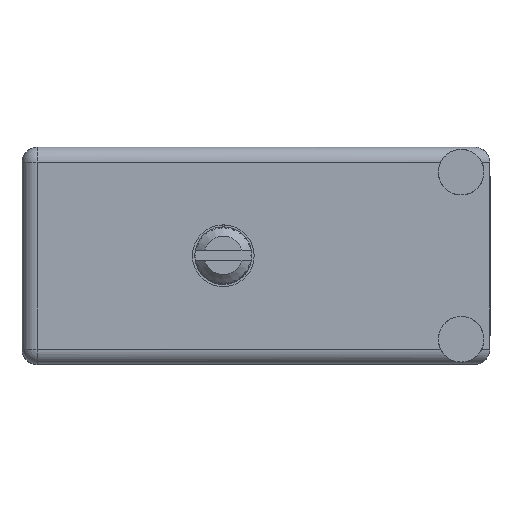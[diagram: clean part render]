
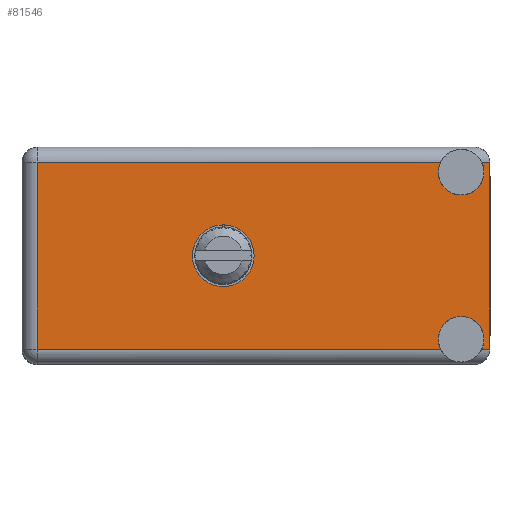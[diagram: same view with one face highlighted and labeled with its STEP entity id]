
A CAD part, top view. The second image highlights one B-rep face of the part: STEP entity #81546.
In plain terms, the highlighted face is planar.
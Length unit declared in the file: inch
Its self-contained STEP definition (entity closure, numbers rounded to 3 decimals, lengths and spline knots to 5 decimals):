
#1102 = EDGE_LOOP ( 'NONE', ( #109759, #47363 ) ) ;
#2539 = ORIENTED_EDGE ( 'NONE', *, *, #103446, .T. ) ;
#3104 = EDGE_CURVE ( 'NONE', #85294, #27077, #30411, .T. ) ;
#4047 = DIRECTION ( 'NONE',  ( 0., 1., 0. ) ) ;
#4627 = CARTESIAN_POINT ( 'NONE',  ( 1.37741, 0.906, -0.05 ) ) ;
#10379 = LINE ( 'NONE', #58055, #128065 ) ;
#10570 = VERTEX_POINT ( 'NONE', #101009 ) ;
#13580 = AXIS2_PLACEMENT_3D ( 'NONE', #35448, #127387, #113257 ) ;
#13898 = VERTEX_POINT ( 'NONE', #93714 ) ;
#14114 = LINE ( 'NONE', #29586, #66838 ) ;
#20758 = EDGE_CURVE ( 'NONE', #189943, #94466, #188819, .T. ) ;
#22841 = CARTESIAN_POINT ( 'NONE',  ( 1.445, 0.906, -0.0825 ) ) ;
#23525 = CARTESIAN_POINT ( 'NONE',  ( 0.6625, 0.906, -0.459 ) ) ;
#24242 = CARTESIAN_POINT ( 'NONE',  ( 0.05, 0.906, -0.05 ) ) ;
#24729 = AXIS2_PLACEMENT_3D ( 'NONE', #22841, #69061, #100625 ) ;
#26307 = DIRECTION ( 'NONE',  ( 0., 0., 1. ) ) ;
#26324 = VERTEX_POINT ( 'NONE', #43488 ) ;
#27077 = VERTEX_POINT ( 'NONE', #24242 ) ;
#28714 = CARTESIAN_POINT ( 'NONE',  ( 0.6625, 0.906, -0.3575 ) ) ;
#29586 = CARTESIAN_POINT ( 'NONE',  ( 0., 0.906, -0.665 ) ) ;
#29957 = DIRECTION ( 'NONE',  ( 0., 0., 1. ) ) ;
#30411 = LINE ( 'NONE', #153032, #179281 ) ;
#32567 = VECTOR ( 'NONE', #26307, 39.37008 ) ;
#35448 = CARTESIAN_POINT ( 'NONE',  ( 0., 0.906, -0.715 ) ) ;
#39727 = LINE ( 'NONE', #88672, #32567 ) ;
#41626 = LINE ( 'NONE', #135473, #92058 ) ;
#41922 = AXIS2_PLACEMENT_3D ( 'NONE', #50361, #4047, #111419 ) ;
#43488 = CARTESIAN_POINT ( 'NONE',  ( 1.37741, 0.906, -0.665 ) ) ;
#47363 = ORIENTED_EDGE ( 'NONE', *, *, #20758, .F. ) ;
#47714 = VECTOR ( 'NONE', #191046, 39.37008 ) ;
#48165 = CIRCLE ( 'NONE', #172847, 0.075 ) ;
#49745 = EDGE_LOOP ( 'NONE', ( #53296, #56450, #165921, #2539, #165619, #97613, #139843, #77111, #56733, #187386 ) ) ;
#50361 = CARTESIAN_POINT ( 'NONE',  ( 1.445, 0.906, -0.6325 ) ) ;
#52321 = DIRECTION ( 'NONE',  ( 0., 1., 0. ) ) ;
#52569 = CARTESIAN_POINT ( 'NONE',  ( 0.6625, 0.906, -0.3575 ) ) ;
#53296 = ORIENTED_EDGE ( 'NONE', *, *, #149624, .T. ) ;
#53889 = DIRECTION ( 'NONE',  ( 0., 0., 1. ) ) ;
#56450 = ORIENTED_EDGE ( 'NONE', *, *, #176888, .F. ) ;
#56733 = ORIENTED_EDGE ( 'NONE', *, *, #111920, .T. ) ;
#58055 = CARTESIAN_POINT ( 'NONE',  ( 1.539, 0.906, -0.05 ) ) ;
#64475 = CIRCLE ( 'NONE', #177485, 0.075 ) ;
#65709 = VERTEX_POINT ( 'NONE', #121247 ) ;
#66838 = VECTOR ( 'NONE', #76492, 39.37008 ) ;
#69061 = DIRECTION ( 'NONE',  ( 0., 1., 0. ) ) ;
#73079 = CARTESIAN_POINT ( 'NONE',  ( 0.6625, 0.906, -0.256 ) ) ;
#74362 = VERTEX_POINT ( 'NONE', #195846 ) ;
#74920 = DIRECTION ( 'NONE',  ( 0., 0., 1. ) ) ;
#75015 = EDGE_CURVE ( 'NONE', #74362, #65709, #39727, .T. ) ;
#76492 = DIRECTION ( 'NONE',  ( -1., 0., 0. ) ) ;
#77111 = ORIENTED_EDGE ( 'NONE', *, *, #189180, .F. ) ;
#77272 = EDGE_CURVE ( 'NONE', #74362, #10570, #41626, .T. ) ;
#81546 = ADVANCED_FACE ( 'NONE', ( #185112, #103423 ), #173097, .T. ) ;
#82005 = CIRCLE ( 'NONE', #41922, 0.075 ) ;
#82099 = DIRECTION ( 'NONE',  ( 0., 1., 0. ) ) ;
#84434 = CARTESIAN_POINT ( 'NONE',  ( 1.51259, 0.906, -0.05 ) ) ;
#85294 = VERTEX_POINT ( 'NONE', #161338 ) ;
#88672 = CARTESIAN_POINT ( 'NONE',  ( 1.539, 0.906, 0. ) ) ;
#89063 = DIRECTION ( 'NONE',  ( 0., 1., 0. ) ) ;
#92058 = VECTOR ( 'NONE', #107224, 39.37008 ) ;
#93714 = CARTESIAN_POINT ( 'NONE',  ( 1.445, 0.906, -0.1575 ) ) ;
#94466 = VERTEX_POINT ( 'NONE', #73079 ) ;
#97329 = CARTESIAN_POINT ( 'NONE',  ( 1.445, 0.906, -0.6325 ) ) ;
#97613 = ORIENTED_EDGE ( 'NONE', *, *, #77272, .T. ) ;
#100625 = DIRECTION ( 'NONE',  ( 0., 0., 1. ) ) ;
#101009 = CARTESIAN_POINT ( 'NONE',  ( 1.51259, 0.906, -0.665 ) ) ;
#102920 = AXIS2_PLACEMENT_3D ( 'NONE', #28714, #89063, #74920 ) ;
#103423 = FACE_OUTER_BOUND ( 'NONE', #49745, .T. ) ;
#103446 = EDGE_CURVE ( 'NONE', #133964, #65709, #10379, .T. ) ;
#107224 = DIRECTION ( 'NONE',  ( -1., 0., 0. ) ) ;
#109759 = ORIENTED_EDGE ( 'NONE', *, *, #182380, .F. ) ;
#111419 = DIRECTION ( 'NONE',  ( 0., 0., 1. ) ) ;
#111920 = EDGE_CURVE ( 'NONE', #26324, #85294, #14114, .T. ) ;
#113257 = DIRECTION ( 'NONE',  ( 0., 0., 1. ) ) ;
#115111 = CARTESIAN_POINT ( 'NONE',  ( 1.539, 0.906, -0.05 ) ) ;
#121247 = CARTESIAN_POINT ( 'NONE',  ( 1.539, 0.906, -0.05 ) ) ;
#121875 = CARTESIAN_POINT ( 'NONE',  ( 1.445, 0.906, -0.0825 ) ) ;
#127387 = DIRECTION ( 'NONE',  ( 0., 1., 0. ) ) ;
#128065 = VECTOR ( 'NONE', #151381, 39.37008 ) ;
#129388 = LINE ( 'NONE', #115111, #47714 ) ;
#130150 = DIRECTION ( 'NONE',  ( 0., 0., 1. ) ) ;
#133964 = VERTEX_POINT ( 'NONE', #84434 ) ;
#135473 = CARTESIAN_POINT ( 'NONE',  ( 0., 0.906, -0.665 ) ) ;
#139115 = CIRCLE ( 'NONE', #24729, 0.075 ) ;
#139843 = ORIENTED_EDGE ( 'NONE', *, *, #195028, .F. ) ;
#139955 = DIRECTION ( 'NONE',  ( 0., 1., 0. ) ) ;
#147233 = EDGE_CURVE ( 'NONE', #133964, #13898, #139115, .T. ) ;
#149624 = EDGE_CURVE ( 'NONE', #27077, #184970, #129388, .T. ) ;
#151381 = DIRECTION ( 'NONE',  ( 1., 0., 0. ) ) ;
#153032 = CARTESIAN_POINT ( 'NONE',  ( 0.05, 0.906, -0.715 ) ) ;
#155912 = VERTEX_POINT ( 'NONE', #156423 ) ;
#156423 = CARTESIAN_POINT ( 'NONE',  ( 1.445, 0.906, -0.5575 ) ) ;
#161338 = CARTESIAN_POINT ( 'NONE',  ( 0.05, 0.906, -0.665 ) ) ;
#165619 = ORIENTED_EDGE ( 'NONE', *, *, #75015, .F. ) ;
#165921 = ORIENTED_EDGE ( 'NONE', *, *, #147233, .F. ) ;
#167804 = DIRECTION ( 'NONE',  ( 0., 0., 1. ) ) ;
#167972 = CIRCLE ( 'NONE', #175711, 0.1015 ) ;
#172847 = AXIS2_PLACEMENT_3D ( 'NONE', #97329, #52321, #130150 ) ;
#173097 = PLANE ( 'NONE',  #13580 ) ;
#175711 = AXIS2_PLACEMENT_3D ( 'NONE', #52569, #82099, #53889 ) ;
#176888 = EDGE_CURVE ( 'NONE', #13898, #184970, #64475, .T. ) ;
#177485 = AXIS2_PLACEMENT_3D ( 'NONE', #121875, #139955, #29957 ) ;
#179281 = VECTOR ( 'NONE', #167804, 39.37008 ) ;
#182380 = EDGE_CURVE ( 'NONE', #94466, #189943, #167972, .T. ) ;
#184970 = VERTEX_POINT ( 'NONE', #4627 ) ;
#185112 = FACE_BOUND ( 'NONE', #1102, .T. ) ;
#187386 = ORIENTED_EDGE ( 'NONE', *, *, #3104, .T. ) ;
#188819 = CIRCLE ( 'NONE', #102920, 0.1015 ) ;
#189180 = EDGE_CURVE ( 'NONE', #26324, #155912, #82005, .T. ) ;
#189943 = VERTEX_POINT ( 'NONE', #23525 ) ;
#191046 = DIRECTION ( 'NONE',  ( 1., 0., 0. ) ) ;
#195028 = EDGE_CURVE ( 'NONE', #155912, #10570, #48165, .T. ) ;
#195846 = CARTESIAN_POINT ( 'NONE',  ( 1.539, 0.906, -0.665 ) ) ;
